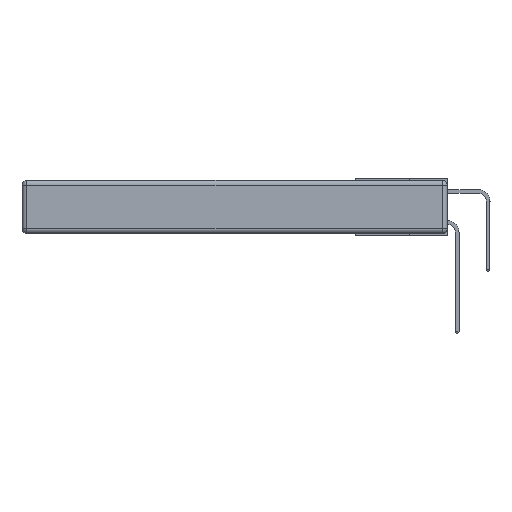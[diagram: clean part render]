
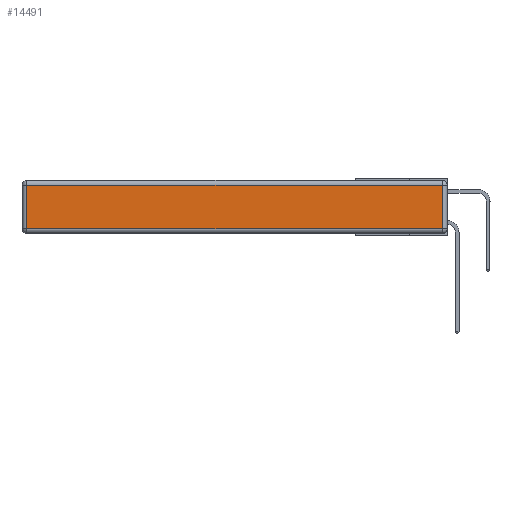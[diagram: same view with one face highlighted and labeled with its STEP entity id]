
A CAD part, left-side view. The second image highlights one B-rep face of the part: STEP entity #14491.
In plain terms, the highlighted planar face has unit normal (-1, 0, 0).
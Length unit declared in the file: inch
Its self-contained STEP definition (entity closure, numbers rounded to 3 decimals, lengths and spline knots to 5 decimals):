
#526 = EDGE_CURVE ( 'NONE', #5730, #6187, #4873, .T. ) ;
#1434 = DIRECTION ( 'NONE',  ( 0., -1., 0. ) ) ;
#1707 = CARTESIAN_POINT ( 'NONE',  ( 0., 2.72, -0.03 ) ) ;
#2469 = VERTEX_POINT ( 'NONE', #3827 ) ;
#3226 = ORIENTED_EDGE ( 'NONE', *, *, #9142, .T. ) ;
#3676 = CARTESIAN_POINT ( 'NONE',  ( 0., 0.03, -0.313 ) ) ;
#3827 = CARTESIAN_POINT ( 'NONE',  ( 0., 0.03, -0.03 ) ) ;
#4193 = EDGE_CURVE ( 'NONE', #2469, #11704, #6858, .T. ) ;
#4248 = AXIS2_PLACEMENT_3D ( 'NONE', #11297, #13947, #12668 ) ;
#4751 = FACE_OUTER_BOUND ( 'NONE', #12600, .T. ) ;
#4873 = LINE ( 'NONE', #5288, #8573 ) ;
#5288 = CARTESIAN_POINT ( 'NONE',  ( 0., 0., -0.313 ) ) ;
#5730 = VERTEX_POINT ( 'NONE', #12088 ) ;
#6187 = VERTEX_POINT ( 'NONE', #3676 ) ;
#6295 = LINE ( 'NONE', #16924, #8932 ) ;
#6858 = LINE ( 'NONE', #9160, #16364 ) ;
#7822 = LINE ( 'NONE', #14773, #15479 ) ;
#8573 = VECTOR ( 'NONE', #1434, 39.37008 ) ;
#8932 = VECTOR ( 'NONE', #12968, 39.37008 ) ;
#9142 = EDGE_CURVE ( 'NONE', #11704, #5730, #6295, .T. ) ;
#9160 = CARTESIAN_POINT ( 'NONE',  ( 0., 2.75, -0.03 ) ) ;
#9961 = PLANE ( 'NONE',  #4248 ) ;
#10946 = ORIENTED_EDGE ( 'NONE', *, *, #13252, .T. ) ;
#11297 = CARTESIAN_POINT ( 'NONE',  ( 0., 0., -0.343 ) ) ;
#11704 = VERTEX_POINT ( 'NONE', #1707 ) ;
#12088 = CARTESIAN_POINT ( 'NONE',  ( 0., 2.72, -0.313 ) ) ;
#12600 = EDGE_LOOP ( 'NONE', ( #14267, #10946, #14759, #3226 ) ) ;
#12668 = DIRECTION ( 'NONE',  ( 0., 0., 1. ) ) ;
#12968 = DIRECTION ( 'NONE',  ( 0., 0., -1. ) ) ;
#13252 = EDGE_CURVE ( 'NONE', #6187, #2469, #7822, .T. ) ;
#13947 = DIRECTION ( 'NONE',  ( -1., 0., 0. ) ) ;
#14267 = ORIENTED_EDGE ( 'NONE', *, *, #526, .T. ) ;
#14417 = DIRECTION ( 'NONE',  ( 0., 1., 0. ) ) ;
#14491 = ADVANCED_FACE ( 'NONE', ( #4751 ), #9961, .T. ) ;
#14759 = ORIENTED_EDGE ( 'NONE', *, *, #4193, .T. ) ;
#14773 = CARTESIAN_POINT ( 'NONE',  ( 0., 0.03, -0.343 ) ) ;
#15479 = VECTOR ( 'NONE', #15842, 39.37008 ) ;
#15842 = DIRECTION ( 'NONE',  ( 0., 0., 1. ) ) ;
#16364 = VECTOR ( 'NONE', #14417, 39.37008 ) ;
#16924 = CARTESIAN_POINT ( 'NONE',  ( 0., 2.72, -0.343 ) ) ;
